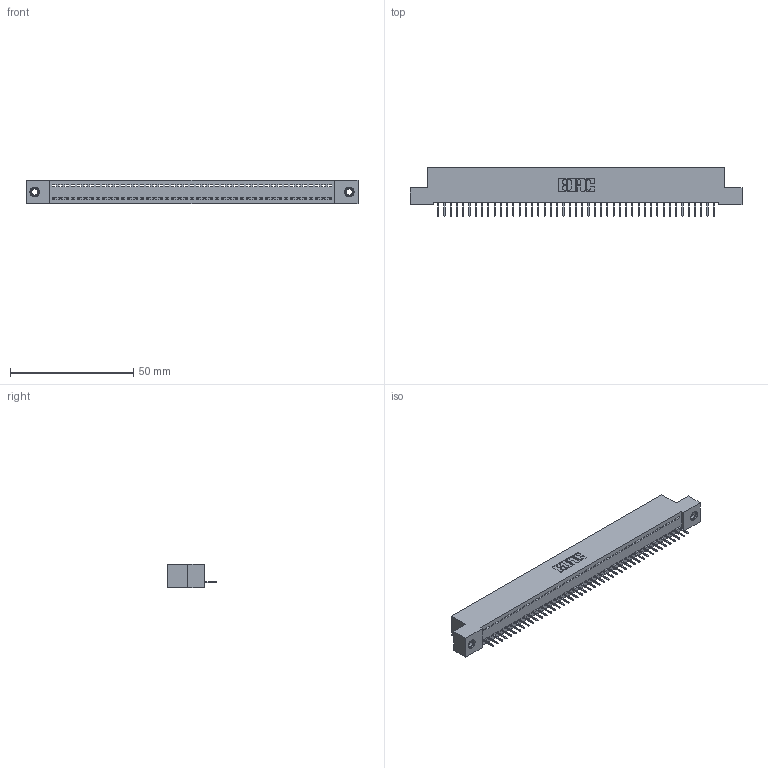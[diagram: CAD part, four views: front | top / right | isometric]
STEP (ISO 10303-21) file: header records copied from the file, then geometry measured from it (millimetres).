
FILE_DESCRIPTION (( 'STEP AP203' ), '1' );
FILE_NAME ('342-045-524-107.STEP', '2018-08-12T15:22:16', ( '' ), ( '' ), 'SwSTEP 2.0', 'SolidWorks 2016', '' );
FILE_SCHEMA (( 'CONFIG_CONTROL_DESIGN' ));
Length unit declared in the file: inch
Products named in the file (4): 342 Part_TI; 345-292-001_345-293-124; 345-250-001_345-250-005-103; 342-045-524-107
Assembly tree (48 placements, depth 2):
  342-045-524-107
    342 Part_TI
    345-292-001_345-293-124  x45
    345-250-001_345-250-005-103  x2
Bounding box: 134.62 x 19.69 x 9.4 mm (x, y, z)
Volume: 11624.1 mm3; surface area: 16605.5 mm2
Topology: 48 solids, 48 shells, 2960 faces, 8535 edges, 5502 vertices
Faces by surface type: plane 2258, cylinder 686, cone 12, torus 4
Entity records: 28250 total; most frequent: CARTESIAN_POINT 4852, ORIENTED_EDGE 4826, DIRECTION 4121, EDGE_CURVE 2413, LINE 2269, VECTOR 2269, VERTEX_POINT 1600, AXIS2_PLACEMENT_3D 926
